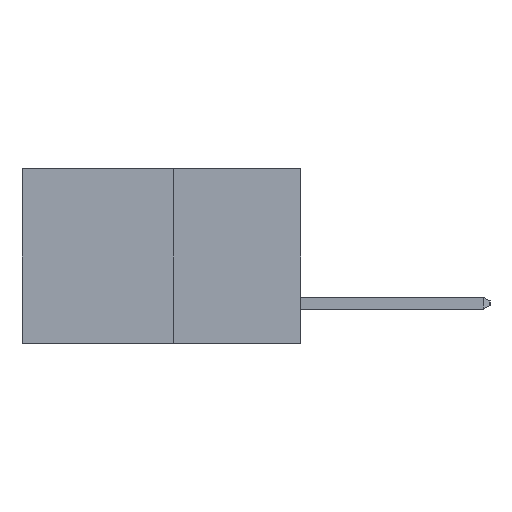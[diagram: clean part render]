
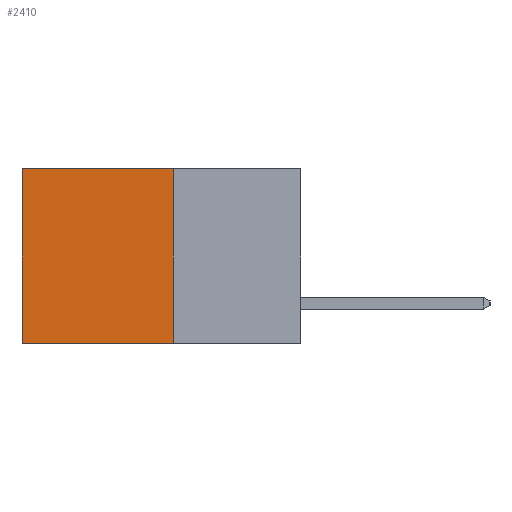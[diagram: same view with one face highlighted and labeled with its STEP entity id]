
A CAD part, left-side view. The second image highlights one B-rep face of the part: STEP entity #2410.
In plain terms, the highlighted planar face has unit normal (-1, 0, 0).
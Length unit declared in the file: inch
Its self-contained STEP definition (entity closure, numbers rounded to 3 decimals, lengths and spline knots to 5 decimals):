
#919 = DIRECTION ( 'NONE',  ( 0., 1., 0. ) ) ;
#1008 = LINE ( 'NONE', #4825, #5322 ) ;
#1027 = DIRECTION ( 'NONE',  ( 0., 0., -1. ) ) ;
#1153 = FACE_OUTER_BOUND ( 'NONE', #6277, .T. ) ;
#1209 = EDGE_CURVE ( 'NONE', #9882, #3636, #1869, .T. ) ;
#1258 = EDGE_CURVE ( 'NONE', #3636, #6188, #8162, .T. ) ;
#1845 = CARTESIAN_POINT ( 'NONE',  ( 0.277, 0.59, 0. ) ) ;
#1869 = LINE ( 'NONE', #9621, #6274 ) ;
#2161 = LINE ( 'NONE', #5010, #8439 ) ;
#2410 = ADVANCED_FACE ( 'NONE', ( #1153 ), #5326, .F. ) ;
#2423 = VERTEX_POINT ( 'NONE', #1845 ) ;
#2694 = EDGE_CURVE ( 'NONE', #9882, #2423, #1008, .T. ) ;
#3636 = VERTEX_POINT ( 'NONE', #7206 ) ;
#4610 = ORIENTED_EDGE ( 'NONE', *, *, #1209, .F. ) ;
#4749 = CARTESIAN_POINT ( 'NONE',  ( 0.277, 0.27, -0.37 ) ) ;
#4825 = CARTESIAN_POINT ( 'NONE',  ( 0.277, 0.27, 0. ) ) ;
#5010 = CARTESIAN_POINT ( 'NONE',  ( 0.277, 0.59, -0.37 ) ) ;
#5045 = DIRECTION ( 'NONE',  ( 0., 0., -1. ) ) ;
#5287 = EDGE_CURVE ( 'NONE', #2423, #6188, #2161, .T. ) ;
#5322 = VECTOR ( 'NONE', #919, 39.37008 ) ;
#5326 = PLANE ( 'NONE',  #6257 ) ;
#5810 = VECTOR ( 'NONE', #7665, 39.37008 ) ;
#6188 = VERTEX_POINT ( 'NONE', #10548 ) ;
#6257 = AXIS2_PLACEMENT_3D ( 'NONE', #4749, #9446, #1027 ) ;
#6274 = VECTOR ( 'NONE', #9289, 39.37008 ) ;
#6277 = EDGE_LOOP ( 'NONE', ( #8047, #10592, #4610, #9045 ) ) ;
#6652 = CARTESIAN_POINT ( 'NONE',  ( 0.277, 0.27, -0.37 ) ) ;
#7206 = CARTESIAN_POINT ( 'NONE',  ( 0.277, 0.27, -0.37 ) ) ;
#7665 = DIRECTION ( 'NONE',  ( 0., 1., 0. ) ) ;
#8047 = ORIENTED_EDGE ( 'NONE', *, *, #5287, .T. ) ;
#8162 = LINE ( 'NONE', #6652, #5810 ) ;
#8439 = VECTOR ( 'NONE', #5045, 39.37008 ) ;
#8524 = CARTESIAN_POINT ( 'NONE',  ( 0.277, 0.27, 0. ) ) ;
#9045 = ORIENTED_EDGE ( 'NONE', *, *, #2694, .T. ) ;
#9289 = DIRECTION ( 'NONE',  ( 0., 0., -1. ) ) ;
#9446 = DIRECTION ( 'NONE',  ( 1., 0., 0. ) ) ;
#9621 = CARTESIAN_POINT ( 'NONE',  ( 0.277, 0.27, -0.37 ) ) ;
#9882 = VERTEX_POINT ( 'NONE', #8524 ) ;
#10548 = CARTESIAN_POINT ( 'NONE',  ( 0.277, 0.59, -0.37 ) ) ;
#10592 = ORIENTED_EDGE ( 'NONE', *, *, #1258, .F. ) ;
